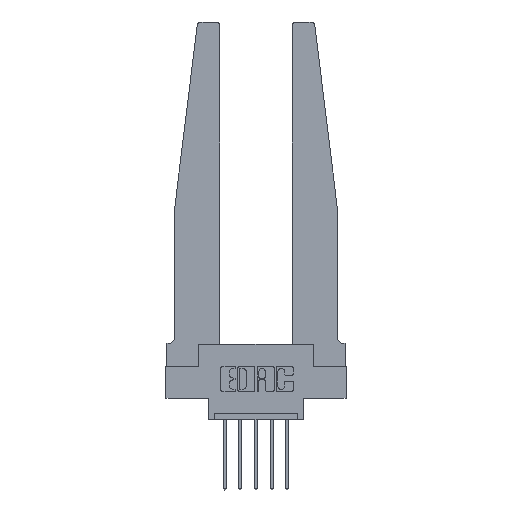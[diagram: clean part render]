
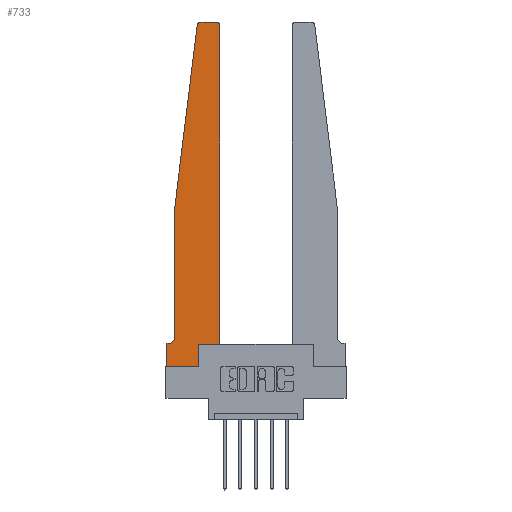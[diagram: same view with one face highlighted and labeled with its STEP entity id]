
A CAD part, top view. The second image highlights one B-rep face of the part: STEP entity #733.
In plain terms, the highlighted planar face has unit normal (0, 0, 1).
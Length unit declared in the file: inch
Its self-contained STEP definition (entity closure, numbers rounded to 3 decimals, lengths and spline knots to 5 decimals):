
#246 = EDGE_CURVE ( 'NONE', #5502, #9087, #7792, .T. ) ;
#416 = EDGE_CURVE ( 'NONE', #13290, #4509, #980, .T. ) ;
#429 = LINE ( 'NONE', #4630, #5880 ) ;
#434 = VERTEX_POINT ( 'NONE', #9280 ) ;
#459 = DIRECTION ( 'NONE',  ( 1., 0., 0. ) ) ;
#568 = ORIENTED_EDGE ( 'NONE', *, *, #12216, .T. ) ;
#615 = DIRECTION ( 'NONE',  ( -1., 0., 0. ) ) ;
#733 = ADVANCED_FACE ( 'NONE', ( #2599 ), #2387, .T. ) ;
#737 = DIRECTION ( 'NONE',  ( -0.122, -0.992, 0. ) ) ;
#980 = LINE ( 'NONE', #5885, #8724 ) ;
#1016 = DIRECTION ( 'NONE',  ( 0., 0., 1. ) ) ;
#1257 = CARTESIAN_POINT ( 'NONE',  ( 0.27653, 2.75, 0.37 ) ) ;
#1315 = DIRECTION ( 'NONE',  ( 0., 1., 0. ) ) ;
#1448 = ORIENTED_EDGE ( 'NONE', *, *, #13193, .T. ) ;
#1456 = CIRCLE ( 'NONE', #8845, 0.05 ) ;
#1604 = VERTEX_POINT ( 'NONE', #8399 ) ;
#1612 = CARTESIAN_POINT ( 'NONE',  ( 0.065, 0.2375, 0.37 ) ) ;
#1827 = CIRCLE ( 'NONE', #3385, 0.03 ) ;
#1936 = DIRECTION ( 'NONE',  ( -1., 0., 0. ) ) ;
#2103 = EDGE_CURVE ( 'NONE', #1604, #13290, #3986, .T. ) ;
#2387 = PLANE ( 'NONE',  #5737 ) ;
#2457 = LINE ( 'NONE', #6625, #7151 ) ;
#2507 = EDGE_CURVE ( 'NONE', #11631, #12948, #429, .T. ) ;
#2599 = FACE_OUTER_BOUND ( 'NONE', #8706, .T. ) ;
#2856 = LINE ( 'NONE', #9137, #5861 ) ;
#3055 = DIRECTION ( 'NONE',  ( 0., 1., 0. ) ) ;
#3114 = ORIENTED_EDGE ( 'NONE', *, *, #9015, .T. ) ;
#3142 = ORIENTED_EDGE ( 'NONE', *, *, #2507, .T. ) ;
#3153 = DIRECTION ( 'NONE',  ( 0., 0., 1. ) ) ;
#3200 = CARTESIAN_POINT ( 'NONE',  ( 0.065, 1.25, 0.37 ) ) ;
#3385 = AXIS2_PLACEMENT_3D ( 'NONE', #10345, #1016, #9318 ) ;
#3501 = DIRECTION ( 'NONE',  ( 1., 0., 0. ) ) ;
#3621 = CARTESIAN_POINT ( 'NONE',  ( 0.015, 0.2375, 0.37 ) ) ;
#3986 = LINE ( 'NONE', #10053, #9297 ) ;
#4263 = ORIENTED_EDGE ( 'NONE', *, *, #4920, .T. ) ;
#4313 = CARTESIAN_POINT ( 'NONE',  ( 0.425, 0.18, 0.37 ) ) ;
#4405 = CARTESIAN_POINT ( 'NONE',  ( 0., 0.1875, 0.37 ) ) ;
#4477 = ORIENTED_EDGE ( 'NONE', *, *, #246, .T. ) ;
#4509 = VERTEX_POINT ( 'NONE', #1612 ) ;
#4630 = CARTESIAN_POINT ( 'NONE',  ( 0.065, 0.1875, 0.37 ) ) ;
#4920 = EDGE_CURVE ( 'NONE', #10802, #1604, #1827, .T. ) ;
#5179 = DIRECTION ( 'NONE',  ( 0., -1., 0. ) ) ;
#5424 = ORIENTED_EDGE ( 'NONE', *, *, #7567, .T. ) ;
#5495 = VECTOR ( 'NONE', #1315, 39.37008 ) ;
#5502 = VERTEX_POINT ( 'NONE', #12095 ) ;
#5653 = CARTESIAN_POINT ( 'NONE',  ( 0., 0.1875, 0.37 ) ) ;
#5737 = AXIS2_PLACEMENT_3D ( 'NONE', #5653, #9781, #459 ) ;
#5861 = VECTOR ( 'NONE', #11014, 39.37008 ) ;
#5880 = VECTOR ( 'NONE', #615, 39.37008 ) ;
#5885 = CARTESIAN_POINT ( 'NONE',  ( 0.065, 1.25, 0.37 ) ) ;
#6625 = CARTESIAN_POINT ( 'NONE',  ( 0., 0., 0.37 ) ) ;
#6638 = VECTOR ( 'NONE', #11169, 39.37008 ) ;
#6951 = CARTESIAN_POINT ( 'NONE',  ( 0.425, 0.18, 0.37 ) ) ;
#7030 = VECTOR ( 'NONE', #3055, 39.37008 ) ;
#7151 = VECTOR ( 'NONE', #3501, 39.37008 ) ;
#7267 = LINE ( 'NONE', #11360, #7030 ) ;
#7567 = EDGE_CURVE ( 'NONE', #7575, #9740, #7267, .T. ) ;
#7575 = VERTEX_POINT ( 'NONE', #4313 ) ;
#7723 = CIRCLE ( 'NONE', #13343, 0.03 ) ;
#7792 = LINE ( 'NONE', #9688, #5495 ) ;
#8152 = LINE ( 'NONE', #6951, #6638 ) ;
#8346 = EDGE_CURVE ( 'NONE', #9087, #7575, #8152, .T. ) ;
#8399 = CARTESIAN_POINT ( 'NONE',  ( 0.24675, 2.72367, 0.37 ) ) ;
#8429 = CARTESIAN_POINT ( 'NONE',  ( 0.395, 2.72, 0.37 ) ) ;
#8706 = EDGE_LOOP ( 'NONE', ( #1448, #4263, #11265, #10723, #10121, #3142, #568, #11710, #4477, #13134, #5424, #3114 ) ) ;
#8724 = VECTOR ( 'NONE', #5179, 39.37008 ) ;
#8845 = AXIS2_PLACEMENT_3D ( 'NONE', #3621, #13160, #11213 ) ;
#9015 = EDGE_CURVE ( 'NONE', #9740, #434, #7723, .T. ) ;
#9087 = VERTEX_POINT ( 'NONE', #11291 ) ;
#9137 = CARTESIAN_POINT ( 'NONE',  ( 0., 0., 0.37 ) ) ;
#9280 = CARTESIAN_POINT ( 'NONE',  ( 0.395, 2.75, 0.37 ) ) ;
#9297 = VECTOR ( 'NONE', #737, 39.37008 ) ;
#9318 = DIRECTION ( 'NONE',  ( 1., 0., 0. ) ) ;
#9455 = DIRECTION ( 'NONE',  ( 1., 0., 0. ) ) ;
#9688 = CARTESIAN_POINT ( 'NONE',  ( 0.2605, 0.18, 0.37 ) ) ;
#9740 = VERTEX_POINT ( 'NONE', #10164 ) ;
#9781 = DIRECTION ( 'NONE',  ( 0., 0., 1. ) ) ;
#10053 = CARTESIAN_POINT ( 'NONE',  ( 0.065, 1.25, 0.37 ) ) ;
#10121 = ORIENTED_EDGE ( 'NONE', *, *, #10717, .T. ) ;
#10164 = CARTESIAN_POINT ( 'NONE',  ( 0.425, 2.72, 0.37 ) ) ;
#10190 = VECTOR ( 'NONE', #1936, 39.37008 ) ;
#10345 = CARTESIAN_POINT ( 'NONE',  ( 0.27653, 2.72, 0.37 ) ) ;
#10529 = CARTESIAN_POINT ( 'NONE',  ( 0., 0., 0.37 ) ) ;
#10717 = EDGE_CURVE ( 'NONE', #4509, #11631, #1456, .T. ) ;
#10723 = ORIENTED_EDGE ( 'NONE', *, *, #416, .T. ) ;
#10802 = VERTEX_POINT ( 'NONE', #1257 ) ;
#10840 = CARTESIAN_POINT ( 'NONE',  ( 0.015, 0.1875, 0.37 ) ) ;
#11014 = DIRECTION ( 'NONE',  ( 0., -1., 0. ) ) ;
#11169 = DIRECTION ( 'NONE',  ( 1., 0., 0. ) ) ;
#11213 = DIRECTION ( 'NONE',  ( -1., 0., 0. ) ) ;
#11265 = ORIENTED_EDGE ( 'NONE', *, *, #2103, .T. ) ;
#11291 = CARTESIAN_POINT ( 'NONE',  ( 0.2605, 0.18, 0.37 ) ) ;
#11304 = CARTESIAN_POINT ( 'NONE',  ( 0.25, 2.75, 0.37 ) ) ;
#11360 = CARTESIAN_POINT ( 'NONE',  ( 0.425, 0.18, 0.37 ) ) ;
#11440 = LINE ( 'NONE', #11304, #10190 ) ;
#11631 = VERTEX_POINT ( 'NONE', #10840 ) ;
#11710 = ORIENTED_EDGE ( 'NONE', *, *, #12931, .T. ) ;
#12095 = CARTESIAN_POINT ( 'NONE',  ( 0.2605, 0., 0.37 ) ) ;
#12216 = EDGE_CURVE ( 'NONE', #12948, #12509, #2856, .T. ) ;
#12509 = VERTEX_POINT ( 'NONE', #10529 ) ;
#12931 = EDGE_CURVE ( 'NONE', #12509, #5502, #2457, .T. ) ;
#12948 = VERTEX_POINT ( 'NONE', #4405 ) ;
#13134 = ORIENTED_EDGE ( 'NONE', *, *, #8346, .T. ) ;
#13160 = DIRECTION ( 'NONE',  ( 0., 0., -1. ) ) ;
#13193 = EDGE_CURVE ( 'NONE', #434, #10802, #11440, .T. ) ;
#13290 = VERTEX_POINT ( 'NONE', #3200 ) ;
#13343 = AXIS2_PLACEMENT_3D ( 'NONE', #8429, #3153, #9455 ) ;
